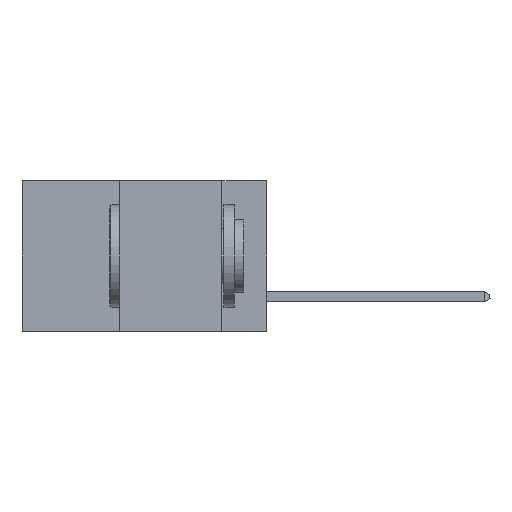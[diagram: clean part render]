
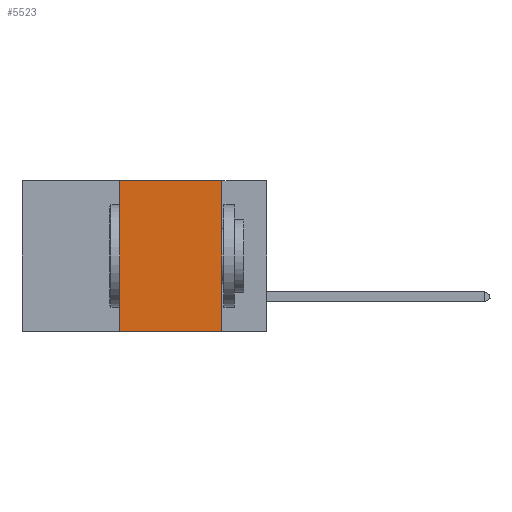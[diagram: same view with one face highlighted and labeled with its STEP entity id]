
A CAD part, left-side view. The second image highlights one B-rep face of the part: STEP entity #5523.
In plain terms, the highlighted planar face has unit normal (-1, 0, 0).
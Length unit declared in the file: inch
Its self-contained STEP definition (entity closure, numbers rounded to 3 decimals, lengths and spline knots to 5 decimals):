
#602 = CARTESIAN_POINT ( 'NONE',  ( 0., 0.36, 0. ) ) ;
#1165 = DIRECTION ( 'NONE',  ( 0., 0., -1. ) ) ;
#1296 = EDGE_LOOP ( 'NONE', ( #4355, #9929, #9055, #8057 ) ) ;
#1431 = VERTEX_POINT ( 'NONE', #4000 ) ;
#1486 = DIRECTION ( 'NONE',  ( 0., -1., 0. ) ) ;
#1548 = DIRECTION ( 'NONE',  ( 1., 0., 0. ) ) ;
#1757 = LINE ( 'NONE', #8006, #9635 ) ;
#2198 = LINE ( 'NONE', #11373, #12781 ) ;
#2490 = VERTEX_POINT ( 'NONE', #6872 ) ;
#2719 = DIRECTION ( 'NONE',  ( 0., 0., -1. ) ) ;
#2834 = VERTEX_POINT ( 'NONE', #602 ) ;
#3942 = DIRECTION ( 'NONE',  ( 0., 0., 1. ) ) ;
#4000 = CARTESIAN_POINT ( 'NONE',  ( 0., 0.11, -0.37 ) ) ;
#4201 = VERTEX_POINT ( 'NONE', #10715 ) ;
#4355 = ORIENTED_EDGE ( 'NONE', *, *, #4772, .F. ) ;
#4772 = EDGE_CURVE ( 'NONE', #4201, #1431, #2198, .T. ) ;
#5101 = CARTESIAN_POINT ( 'NONE',  ( 0., 0.6, -0.37 ) ) ;
#5523 = ADVANCED_FACE ( 'NONE', ( #7442 ), #12798, .F. ) ;
#5946 = LINE ( 'NONE', #10653, #8374 ) ;
#6726 = AXIS2_PLACEMENT_3D ( 'NONE', #7689, #1548, #2719 ) ;
#6867 = LINE ( 'NONE', #5101, #7699 ) ;
#6872 = CARTESIAN_POINT ( 'NONE',  ( 0., 0.36, -0.37 ) ) ;
#7442 = FACE_OUTER_BOUND ( 'NONE', #1296, .T. ) ;
#7689 = CARTESIAN_POINT ( 'NONE',  ( 0., 0.6, 0. ) ) ;
#7699 = VECTOR ( 'NONE', #12462, 39.37008 ) ;
#8006 = CARTESIAN_POINT ( 'NONE',  ( 0., 0.36, 0. ) ) ;
#8057 = ORIENTED_EDGE ( 'NONE', *, *, #8329, .T. ) ;
#8329 = EDGE_CURVE ( 'NONE', #2490, #1431, #6867, .T. ) ;
#8374 = VECTOR ( 'NONE', #1486, 39.37008 ) ;
#9055 = ORIENTED_EDGE ( 'NONE', *, *, #11011, .F. ) ;
#9635 = VECTOR ( 'NONE', #3942, 39.37008 ) ;
#9726 = EDGE_CURVE ( 'NONE', #2834, #4201, #5946, .T. ) ;
#9929 = ORIENTED_EDGE ( 'NONE', *, *, #9726, .F. ) ;
#10653 = CARTESIAN_POINT ( 'NONE',  ( 0., 0.6, 0. ) ) ;
#10715 = CARTESIAN_POINT ( 'NONE',  ( 0., 0.11, 0. ) ) ;
#11011 = EDGE_CURVE ( 'NONE', #2490, #2834, #1757, .T. ) ;
#11373 = CARTESIAN_POINT ( 'NONE',  ( 0., 0.11, 0. ) ) ;
#12462 = DIRECTION ( 'NONE',  ( 0., -1., 0. ) ) ;
#12781 = VECTOR ( 'NONE', #1165, 39.37008 ) ;
#12798 = PLANE ( 'NONE',  #6726 ) ;
